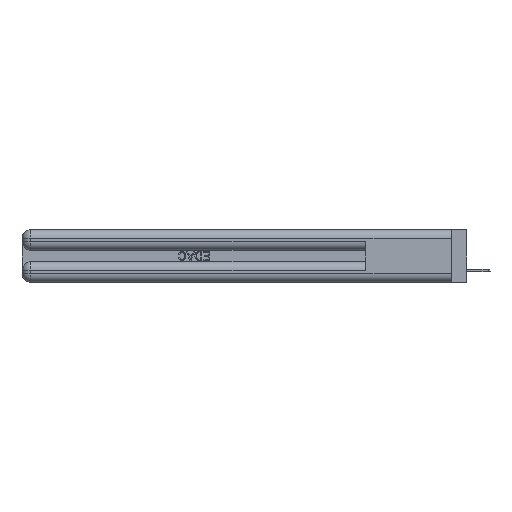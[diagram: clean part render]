
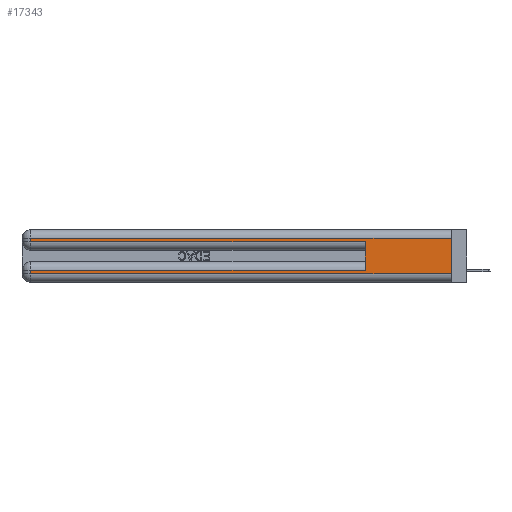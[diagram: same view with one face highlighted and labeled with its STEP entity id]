
A CAD part, left-side view. The second image highlights one B-rep face of the part: STEP entity #17343.
In plain terms, the highlighted planar face has unit normal (-1, 0, 0).
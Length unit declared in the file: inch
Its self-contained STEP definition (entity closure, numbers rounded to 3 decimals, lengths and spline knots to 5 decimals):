
#126 = CARTESIAN_POINT ( 'NONE',  ( 0., 2.94, 0.37 ) ) ;
#391 = CARTESIAN_POINT ( 'NONE',  ( 0., 2.94, 0.06 ) ) ;
#1265 = VERTEX_POINT ( 'NONE', #28873 ) ;
#3045 = DIRECTION ( 'NONE',  ( 0., -1., 0. ) ) ;
#3277 = CARTESIAN_POINT ( 'NONE',  ( 0., 2.94, 0.085 ) ) ;
#3515 = CARTESIAN_POINT ( 'NONE',  ( 0., 0., 0.085 ) ) ;
#3854 = CARTESIAN_POINT ( 'NONE',  ( 0., 0.6, 0.285 ) ) ;
#4378 = LINE ( 'NONE', #39298, #38365 ) ;
#4583 = LINE ( 'NONE', #33431, #34322 ) ;
#4616 = ORIENTED_EDGE ( 'NONE', *, *, #32873, .F. ) ;
#5183 = DIRECTION ( 'NONE',  ( 0., 1., 0. ) ) ;
#5975 = VERTEX_POINT ( 'NONE', #11654 ) ;
#6008 = VECTOR ( 'NONE', #23080, 39.37008 ) ;
#6261 = ORIENTED_EDGE ( 'NONE', *, *, #36875, .T. ) ;
#6487 = DIRECTION ( 'NONE',  ( 0., 0., -1. ) ) ;
#7112 = EDGE_CURVE ( 'NONE', #27605, #33921, #35084, .T. ) ;
#7210 = VECTOR ( 'NONE', #35825, 39.37008 ) ;
#8139 = CARTESIAN_POINT ( 'NONE',  ( 0., 2.94, 0.285 ) ) ;
#8699 = EDGE_CURVE ( 'NONE', #21461, #5975, #23095, .T. ) ;
#9278 = PLANE ( 'NONE',  #41627 ) ;
#9410 = VECTOR ( 'NONE', #3045, 39.37008 ) ;
#9420 = CARTESIAN_POINT ( 'NONE',  ( 0., 0., 0.37 ) ) ;
#11654 = CARTESIAN_POINT ( 'NONE',  ( 0., 2.94, 0.31 ) ) ;
#12404 = CARTESIAN_POINT ( 'NONE',  ( 0., 0., 0.06 ) ) ;
#12430 = CARTESIAN_POINT ( 'NONE',  ( 0., 0., 0.31 ) ) ;
#12615 = DIRECTION ( 'NONE',  ( 1., 0., 0. ) ) ;
#12884 = DIRECTION ( 'NONE',  ( 0., 0., 1. ) ) ;
#13894 = FACE_OUTER_BOUND ( 'NONE', #30157, .T. ) ;
#14394 = ORIENTED_EDGE ( 'NONE', *, *, #39836, .T. ) ;
#14975 = VECTOR ( 'NONE', #6487, 39.37008 ) ;
#15805 = DIRECTION ( 'NONE',  ( 0., 0., -1. ) ) ;
#16027 = DIRECTION ( 'NONE',  ( 0., 0., -1. ) ) ;
#16071 = CARTESIAN_POINT ( 'NONE',  ( 0., 0., 0.37 ) ) ;
#17119 = VERTEX_POINT ( 'NONE', #8139 ) ;
#17343 = ADVANCED_FACE ( 'NONE', ( #13894 ), #9278, .F. ) ;
#18050 = LINE ( 'NONE', #3515, #7210 ) ;
#19549 = VECTOR ( 'NONE', #5183, 39.37008 ) ;
#21461 = VERTEX_POINT ( 'NONE', #12430 ) ;
#21669 = ORIENTED_EDGE ( 'NONE', *, *, #7112, .T. ) ;
#23080 = DIRECTION ( 'NONE',  ( 0., -1., 0. ) ) ;
#23095 = LINE ( 'NONE', #40929, #19549 ) ;
#23898 = LINE ( 'NONE', #35713, #6008 ) ;
#24657 = ORIENTED_EDGE ( 'NONE', *, *, #8699, .T. ) ;
#24932 = ORIENTED_EDGE ( 'NONE', *, *, #41427, .T. ) ;
#26197 = LINE ( 'NONE', #126, #14975 ) ;
#26412 = EDGE_CURVE ( 'NONE', #1265, #42292, #4378, .T. ) ;
#27605 = VERTEX_POINT ( 'NONE', #391 ) ;
#28437 = ORIENTED_EDGE ( 'NONE', *, *, #33015, .T. ) ;
#28873 = CARTESIAN_POINT ( 'NONE',  ( 0., 0.6, 0.085 ) ) ;
#30157 = EDGE_LOOP ( 'NONE', ( #4616, #24657, #24932, #6261, #37080, #28437, #14394, #21669 ) ) ;
#32031 = CARTESIAN_POINT ( 'NONE',  ( 0., 0., 0.06 ) ) ;
#32873 = EDGE_CURVE ( 'NONE', #21461, #33921, #39629, .T. ) ;
#33015 = EDGE_CURVE ( 'NONE', #1265, #33054, #18050, .T. ) ;
#33054 = VERTEX_POINT ( 'NONE', #3277 ) ;
#33431 = CARTESIAN_POINT ( 'NONE',  ( 0., 2.94, 0.37 ) ) ;
#33921 = VERTEX_POINT ( 'NONE', #32031 ) ;
#34322 = VECTOR ( 'NONE', #36620, 39.37008 ) ;
#34463 = VECTOR ( 'NONE', #15805, 39.37008 ) ;
#35084 = LINE ( 'NONE', #12404, #9410 ) ;
#35713 = CARTESIAN_POINT ( 'NONE',  ( 0., 0., 0.285 ) ) ;
#35825 = DIRECTION ( 'NONE',  ( 0., 1., 0. ) ) ;
#36620 = DIRECTION ( 'NONE',  ( 0., 0., -1. ) ) ;
#36875 = EDGE_CURVE ( 'NONE', #17119, #42292, #23898, .T. ) ;
#37080 = ORIENTED_EDGE ( 'NONE', *, *, #26412, .F. ) ;
#38365 = VECTOR ( 'NONE', #12884, 39.37008 ) ;
#39298 = CARTESIAN_POINT ( 'NONE',  ( 0., 0.6, 0.145 ) ) ;
#39629 = LINE ( 'NONE', #16071, #34463 ) ;
#39836 = EDGE_CURVE ( 'NONE', #33054, #27605, #26197, .T. ) ;
#40929 = CARTESIAN_POINT ( 'NONE',  ( 0., 0., 0.31 ) ) ;
#41427 = EDGE_CURVE ( 'NONE', #5975, #17119, #4583, .T. ) ;
#41627 = AXIS2_PLACEMENT_3D ( 'NONE', #9420, #12615, #16027 ) ;
#42292 = VERTEX_POINT ( 'NONE', #3854 ) ;
